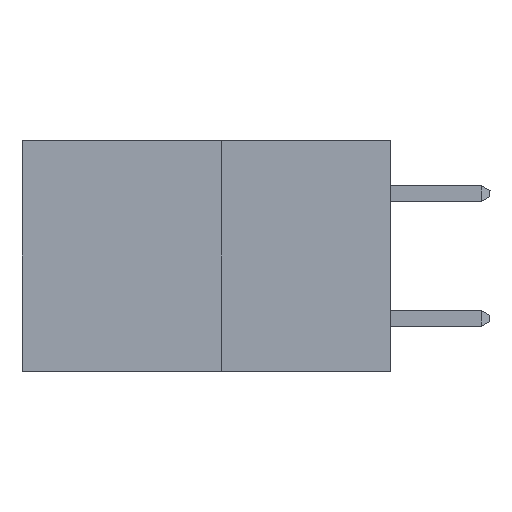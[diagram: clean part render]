
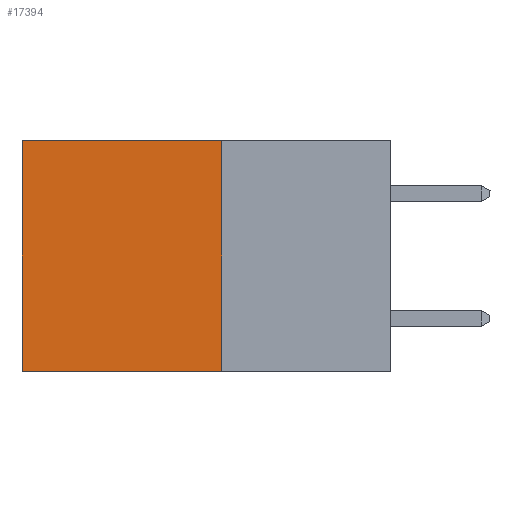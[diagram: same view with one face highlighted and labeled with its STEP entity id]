
A CAD part, left-side view. The second image highlights one B-rep face of the part: STEP entity #17394.
In plain terms, the highlighted planar face has unit normal (-1, 0, 0).
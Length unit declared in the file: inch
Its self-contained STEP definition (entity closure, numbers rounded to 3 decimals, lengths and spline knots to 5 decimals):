
#1013 = DIRECTION ( 'NONE',  ( 0., 0., -1. ) ) ;
#1070 = DIRECTION ( 'NONE',  ( 0., 1., 0. ) ) ;
#1088 = VECTOR ( 'NONE', #17503, 39.37008 ) ;
#1556 = LINE ( 'NONE', #18045, #8665 ) ;
#2039 = LINE ( 'NONE', #5138, #10047 ) ;
#2866 = AXIS2_PLACEMENT_3D ( 'NONE', #17991, #9549, #1013 ) ;
#3427 = VERTEX_POINT ( 'NONE', #15589 ) ;
#4418 = LINE ( 'NONE', #18237, #1088 ) ;
#5138 = CARTESIAN_POINT ( 'NONE',  ( 0.277, 0.27, -0.37 ) ) ;
#5402 = DIRECTION ( 'NONE',  ( 0., 0., -1. ) ) ;
#5721 = EDGE_CURVE ( 'NONE', #3427, #11388, #2039, .T. ) ;
#7373 = VERTEX_POINT ( 'NONE', #7619 ) ;
#7483 = ORIENTED_EDGE ( 'NONE', *, *, #12673, .T. ) ;
#7619 = CARTESIAN_POINT ( 'NONE',  ( 0.277, 0.27, 0. ) ) ;
#7854 = EDGE_CURVE ( 'NONE', #7373, #3427, #4418, .T. ) ;
#8088 = PLANE ( 'NONE',  #2866 ) ;
#8665 = VECTOR ( 'NONE', #1070, 39.37008 ) ;
#9549 = DIRECTION ( 'NONE',  ( 1., 0., 0. ) ) ;
#10047 = VECTOR ( 'NONE', #15357, 39.37008 ) ;
#11388 = VERTEX_POINT ( 'NONE', #12434 ) ;
#12228 = FACE_OUTER_BOUND ( 'NONE', #15655, .T. ) ;
#12434 = CARTESIAN_POINT ( 'NONE',  ( 0.277, 0.59, -0.37 ) ) ;
#12546 = CARTESIAN_POINT ( 'NONE',  ( 0.277, 0.59, -0.37 ) ) ;
#12673 = EDGE_CURVE ( 'NONE', #13693, #11388, #13842, .T. ) ;
#13693 = VERTEX_POINT ( 'NONE', #14478 ) ;
#13842 = LINE ( 'NONE', #12546, #17130 ) ;
#14116 = ORIENTED_EDGE ( 'NONE', *, *, #7854, .F. ) ;
#14478 = CARTESIAN_POINT ( 'NONE',  ( 0.277, 0.59, 0. ) ) ;
#14749 = EDGE_CURVE ( 'NONE', #7373, #13693, #1556, .T. ) ;
#14764 = ORIENTED_EDGE ( 'NONE', *, *, #5721, .F. ) ;
#15357 = DIRECTION ( 'NONE',  ( 0., 1., 0. ) ) ;
#15589 = CARTESIAN_POINT ( 'NONE',  ( 0.277, 0.27, -0.37 ) ) ;
#15655 = EDGE_LOOP ( 'NONE', ( #7483, #14764, #14116, #15896 ) ) ;
#15896 = ORIENTED_EDGE ( 'NONE', *, *, #14749, .T. ) ;
#17130 = VECTOR ( 'NONE', #5402, 39.37008 ) ;
#17394 = ADVANCED_FACE ( 'NONE', ( #12228 ), #8088, .F. ) ;
#17503 = DIRECTION ( 'NONE',  ( 0., 0., -1. ) ) ;
#17991 = CARTESIAN_POINT ( 'NONE',  ( 0.277, 0.27, -0.37 ) ) ;
#18045 = CARTESIAN_POINT ( 'NONE',  ( 0.277, 0.27, 0. ) ) ;
#18237 = CARTESIAN_POINT ( 'NONE',  ( 0.277, 0.27, -0.37 ) ) ;
